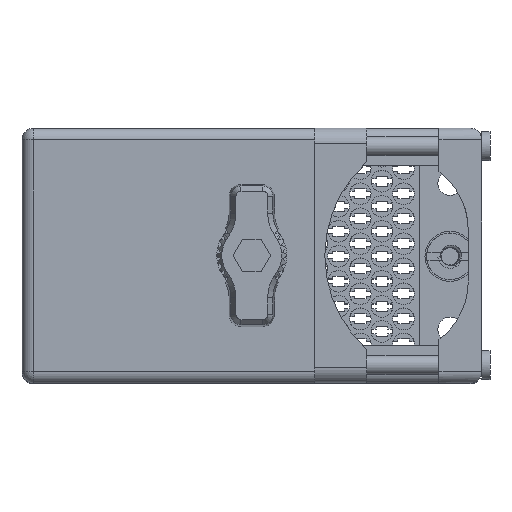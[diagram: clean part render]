
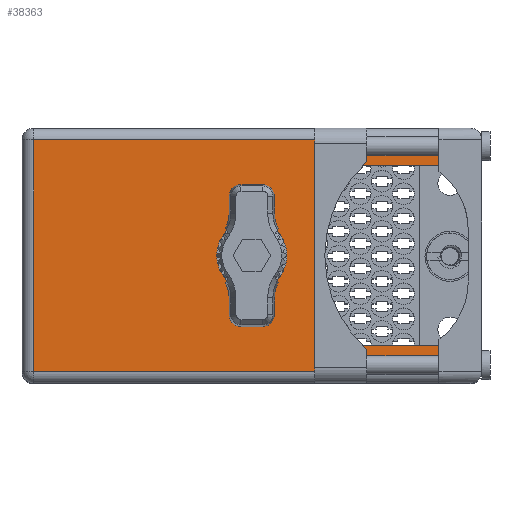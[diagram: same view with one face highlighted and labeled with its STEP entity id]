
A CAD part, top view. The second image highlights one B-rep face of the part: STEP entity #38363.
In plain terms, the highlighted face is planar.
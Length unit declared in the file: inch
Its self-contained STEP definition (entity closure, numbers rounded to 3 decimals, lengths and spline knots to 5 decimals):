
#10 = LINE ( 'NONE', #1301, #55444 ) ;
#1301 = CARTESIAN_POINT ( 'NONE',  ( 1.1215, 1.93, -0.765 ) ) ;
#6135 = DIRECTION ( 'NONE',  ( 0., 0., 1. ) ) ;
#7891 = DIRECTION ( 'NONE',  ( -1., 0., 0. ) ) ;
#8387 = CIRCLE ( 'NONE', #85329, 0.17 ) ;
#9574 = AXIS2_PLACEMENT_3D ( 'NONE', #59079, #66785, #7891 ) ;
#10686 = EDGE_CURVE ( 'NONE', #81535, #48732, #42103, .T. ) ;
#11600 = VERTEX_POINT ( 'NONE', #42503 ) ;
#15680 = DIRECTION ( 'NONE',  ( -1., 0., 0. ) ) ;
#15901 = VERTEX_POINT ( 'NONE', #87062 ) ;
#16091 = ORIENTED_EDGE ( 'NONE', *, *, #10686, .T. ) ;
#19557 = VECTOR ( 'NONE', #53449, 39.37008 ) ;
#21046 = CARTESIAN_POINT ( 'NONE',  ( -1.3775, 1.93, -0.695 ) ) ;
#21075 = VECTOR ( 'NONE', #99643, 39.37008 ) ;
#23723 = CARTESIAN_POINT ( 'NONE',  ( 1.1215, 1.93, -0.54 ) ) ;
#24865 = EDGE_CURVE ( 'NONE', #48732, #80510, #44650, .T. ) ;
#26236 = PLANE ( 'NONE',  #9574 ) ;
#26987 = VERTEX_POINT ( 'NONE', #105952 ) ;
#28810 = CARTESIAN_POINT ( 'NONE',  ( 1.1215, 1.93, -0.765 ) ) ;
#29553 = CARTESIAN_POINT ( 'NONE',  ( 1.1215, 1.93, -0.54 ) ) ;
#29977 = ORIENTED_EDGE ( 'NONE', *, *, #57156, .F. ) ;
#30674 = VERTEX_POINT ( 'NONE', #75576 ) ;
#31977 = DIRECTION ( 'NONE',  ( 1., 0., 0. ) ) ;
#36837 = EDGE_LOOP ( 'NONE', ( #82763, #98910 ) ) ;
#37674 = DIRECTION ( 'NONE',  ( 0., 0., 1. ) ) ;
#38080 = VERTEX_POINT ( 'NONE', #94100 ) ;
#38355 = ORIENTED_EDGE ( 'NONE', *, *, #99877, .F. ) ;
#38363 = ADVANCED_FACE ( 'NONE', ( #94255, #83693 ), #26236, .T. ) ;
#39647 = DIRECTION ( 'NONE',  ( 0., 1., 0. ) ) ;
#41075 = DIRECTION ( 'NONE',  ( 1., 0., 0. ) ) ;
#42103 = LINE ( 'NONE', #21046, #104042 ) ;
#42425 = DIRECTION ( 'NONE',  ( 0., 1., 0. ) ) ;
#42503 = CARTESIAN_POINT ( 'NONE',  ( 1.1215, 1.93, 0.695 ) ) ;
#43024 = EDGE_CURVE ( 'NONE', #59629, #38080, #8387, .T. ) ;
#43519 = EDGE_CURVE ( 'NONE', #80510, #11600, #88716, .T. ) ;
#43647 = LINE ( 'NONE', #49576, #21075 ) ;
#44650 = LINE ( 'NONE', #70355, #19557 ) ;
#46035 = VECTOR ( 'NONE', #41075, 39.37008 ) ;
#48732 = VERTEX_POINT ( 'NONE', #91384 ) ;
#49576 = CARTESIAN_POINT ( 'NONE',  ( 0.4075, 1.93, -0.54 ) ) ;
#50184 = DIRECTION ( 'NONE',  ( 0., 0., 1. ) ) ;
#52111 = EDGE_CURVE ( 'NONE', #38080, #59629, #94524, .T. ) ;
#53449 = DIRECTION ( 'NONE',  ( 0., 0., 1. ) ) ;
#55383 = LINE ( 'NONE', #28810, #68499 ) ;
#55444 = VECTOR ( 'NONE', #68297, 39.37008 ) ;
#57156 = EDGE_CURVE ( 'NONE', #81535, #78049, #55383, .T. ) ;
#57378 = EDGE_LOOP ( 'NONE', ( #81661, #108449, #38355, #95676, #93453, #77931, #29977, #16091 ) ) ;
#59079 = CARTESIAN_POINT ( 'NONE',  ( -1.3775, 1.93, -0.765 ) ) ;
#59629 = VERTEX_POINT ( 'NONE', #65499 ) ;
#62903 = CARTESIAN_POINT ( 'NONE',  ( 1.1215, 1.93, -0.695 ) ) ;
#63891 = AXIS2_PLACEMENT_3D ( 'NONE', #64370, #39647, #6135 ) ;
#64370 = CARTESIAN_POINT ( 'NONE',  ( 0., 1.93, 0. ) ) ;
#65260 = LINE ( 'NONE', #65780, #103509 ) ;
#65499 = CARTESIAN_POINT ( 'NONE',  ( 0., 1.93, 0.17 ) ) ;
#65780 = CARTESIAN_POINT ( 'NONE',  ( 1.1215, 1.93, 0.54 ) ) ;
#66309 = VECTOR ( 'NONE', #31977, 39.37008 ) ;
#66785 = DIRECTION ( 'NONE',  ( 0., 1., 0. ) ) ;
#68297 = DIRECTION ( 'NONE',  ( 0., 0., 1. ) ) ;
#68345 = EDGE_CURVE ( 'NONE', #26987, #78049, #92055, .T. ) ;
#68499 = VECTOR ( 'NONE', #37674, 39.37008 ) ;
#70355 = CARTESIAN_POINT ( 'NONE',  ( -1.3075, 1.93, -0.765 ) ) ;
#71891 = DIRECTION ( 'NONE',  ( -1., 0., 0. ) ) ;
#74377 = EDGE_CURVE ( 'NONE', #30674, #15901, #65260, .T. ) ;
#75040 = CARTESIAN_POINT ( 'NONE',  ( 1.1215, 1.93, 0.695 ) ) ;
#75576 = CARTESIAN_POINT ( 'NONE',  ( 1.1215, 1.93, 0.54 ) ) ;
#77738 = EDGE_CURVE ( 'NONE', #15901, #26987, #43647, .T. ) ;
#77931 = ORIENTED_EDGE ( 'NONE', *, *, #68345, .T. ) ;
#78049 = VERTEX_POINT ( 'NONE', #29553 ) ;
#80510 = VERTEX_POINT ( 'NONE', #108789 ) ;
#81535 = VERTEX_POINT ( 'NONE', #62903 ) ;
#81661 = ORIENTED_EDGE ( 'NONE', *, *, #24865, .T. ) ;
#82763 = ORIENTED_EDGE ( 'NONE', *, *, #43024, .F. ) ;
#83693 = FACE_BOUND ( 'NONE', #36837, .T. ) ;
#85329 = AXIS2_PLACEMENT_3D ( 'NONE', #91764, #42425, #50184 ) ;
#87062 = CARTESIAN_POINT ( 'NONE',  ( 0.4075, 1.93, 0.54 ) ) ;
#88716 = LINE ( 'NONE', #75040, #66309 ) ;
#91384 = CARTESIAN_POINT ( 'NONE',  ( -1.3075, 1.93, -0.695 ) ) ;
#91764 = CARTESIAN_POINT ( 'NONE',  ( 0., 1.93, 0. ) ) ;
#92055 = LINE ( 'NONE', #23723, #46035 ) ;
#93453 = ORIENTED_EDGE ( 'NONE', *, *, #77738, .T. ) ;
#94100 = CARTESIAN_POINT ( 'NONE',  ( 0., 1.93, -0.17 ) ) ;
#94255 = FACE_OUTER_BOUND ( 'NONE', #57378, .T. ) ;
#94524 = CIRCLE ( 'NONE', #63891, 0.17 ) ;
#95676 = ORIENTED_EDGE ( 'NONE', *, *, #74377, .T. ) ;
#98910 = ORIENTED_EDGE ( 'NONE', *, *, #52111, .F. ) ;
#99643 = DIRECTION ( 'NONE',  ( 0., 0., -1. ) ) ;
#99877 = EDGE_CURVE ( 'NONE', #30674, #11600, #10, .T. ) ;
#103509 = VECTOR ( 'NONE', #15680, 39.37008 ) ;
#104042 = VECTOR ( 'NONE', #71891, 39.37008 ) ;
#105952 = CARTESIAN_POINT ( 'NONE',  ( 0.4075, 1.93, -0.54 ) ) ;
#108449 = ORIENTED_EDGE ( 'NONE', *, *, #43519, .T. ) ;
#108789 = CARTESIAN_POINT ( 'NONE',  ( -1.3075, 1.93, 0.695 ) ) ;
